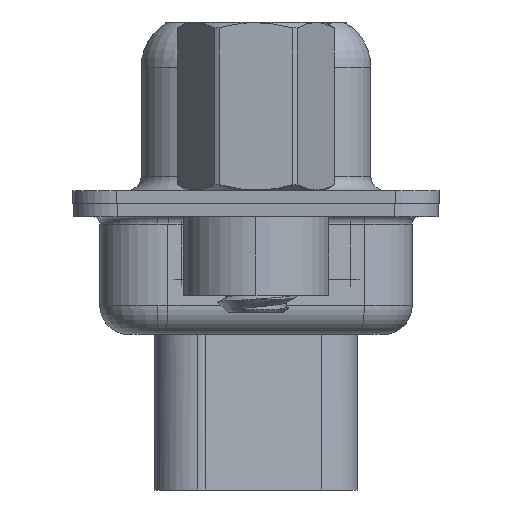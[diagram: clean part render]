
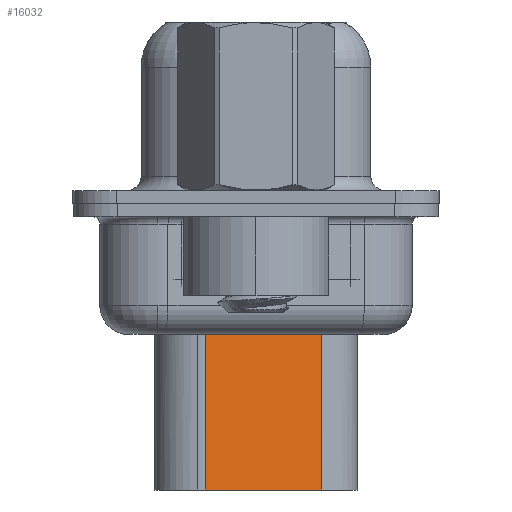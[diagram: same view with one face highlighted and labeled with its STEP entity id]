
A CAD part, left-side view. The second image highlights one B-rep face of the part: STEP entity #16032.
In plain terms, the highlighted planar face has unit normal (-0.985, -0.174, 0).
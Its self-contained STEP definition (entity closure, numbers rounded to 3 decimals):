
#90 = VERTEX_POINT ( 'NONE', #8590 ) ;
#1626 = DIRECTION ( 'NONE',  ( -0.174, 0.985, 0. ) ) ;
#2308 = ORIENTED_EDGE ( 'NONE', *, *, #14520, .F. ) ;
#2433 = EDGE_CURVE ( 'NONE', #6748, #29001, #19044, .T. ) ;
#2720 = ORIENTED_EDGE ( 'NONE', *, *, #19665, .T. ) ;
#3665 = EDGE_CURVE ( 'NONE', #6748, #90, #12392, .T. ) ;
#4523 = DIRECTION ( 'NONE',  ( 0., 0., -1. ) ) ;
#5671 = CARTESIAN_POINT ( 'NONE',  ( 4.524, 1.74, -3.975 ) ) ;
#5894 = VECTOR ( 'NONE', #6855, 1000. ) ;
#6748 = VERTEX_POINT ( 'NONE', #15166 ) ;
#6855 = DIRECTION ( 'NONE',  ( 0., 0., -1. ) ) ;
#7310 = LINE ( 'NONE', #16181, #27675 ) ;
#8590 = CARTESIAN_POINT ( 'NONE',  ( 5.229, -2.26, -9.85 ) ) ;
#8668 = DIRECTION ( 'NONE',  ( 0.174, -0.985, 0. ) ) ;
#10155 = CARTESIAN_POINT ( 'NONE',  ( 4.524, 1.74, -9.85 ) ) ;
#10479 = DIRECTION ( 'NONE',  ( -0.174, 0.985, 0. ) ) ;
#11137 = VECTOR ( 'NONE', #1626, 1000. ) ;
#11194 = ORIENTED_EDGE ( 'NONE', *, *, #2433, .T. ) ;
#12392 = LINE ( 'NONE', #32256, #5894 ) ;
#14230 = FACE_OUTER_BOUND ( 'NONE', #27854, .T. ) ;
#14520 = EDGE_CURVE ( 'NONE', #90, #14918, #30368, .T. ) ;
#14918 = VERTEX_POINT ( 'NONE', #24211 ) ;
#15166 = CARTESIAN_POINT ( 'NONE',  ( 5.229, -2.26, -3.975 ) ) ;
#15393 = AXIS2_PLACEMENT_3D ( 'NONE', #25177, #25548, #8668 ) ;
#16032 = ADVANCED_FACE ( 'NONE', ( #14230 ), #28530, .T. ) ;
#16181 = CARTESIAN_POINT ( 'NONE',  ( 4.524, 1.74, -3.1 ) ) ;
#19044 = LINE ( 'NONE', #35903, #25149 ) ;
#19665 = EDGE_CURVE ( 'NONE', #29001, #14918, #7310, .T. ) ;
#24211 = CARTESIAN_POINT ( 'NONE',  ( 4.524, 1.74, -9.85 ) ) ;
#24615 = ORIENTED_EDGE ( 'NONE', *, *, #3665, .F. ) ;
#25149 = VECTOR ( 'NONE', #10479, 1000. ) ;
#25177 = CARTESIAN_POINT ( 'NONE',  ( 4.524, 1.74, -3.1 ) ) ;
#25548 = DIRECTION ( 'NONE',  ( -0.985, -0.174, 0. ) ) ;
#27675 = VECTOR ( 'NONE', #4523, 1000. ) ;
#27854 = EDGE_LOOP ( 'NONE', ( #24615, #11194, #2720, #2308 ) ) ;
#28530 = PLANE ( 'NONE',  #15393 ) ;
#29001 = VERTEX_POINT ( 'NONE', #5671 ) ;
#30368 = LINE ( 'NONE', #10155, #11137 ) ;
#32256 = CARTESIAN_POINT ( 'NONE',  ( 5.229, -2.26, -3.1 ) ) ;
#35903 = CARTESIAN_POINT ( 'NONE',  ( 4.353, 2.709, -3.975 ) ) ;
